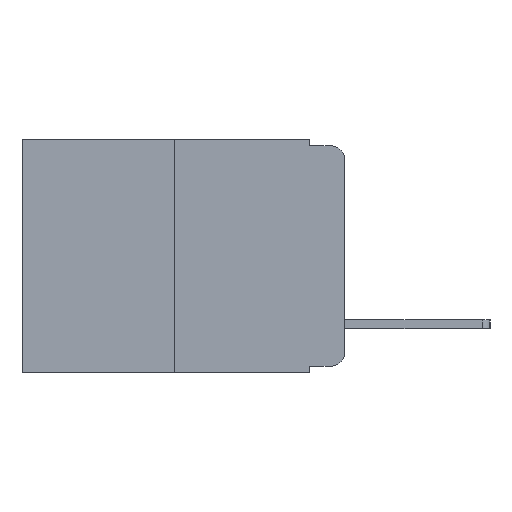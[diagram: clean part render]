
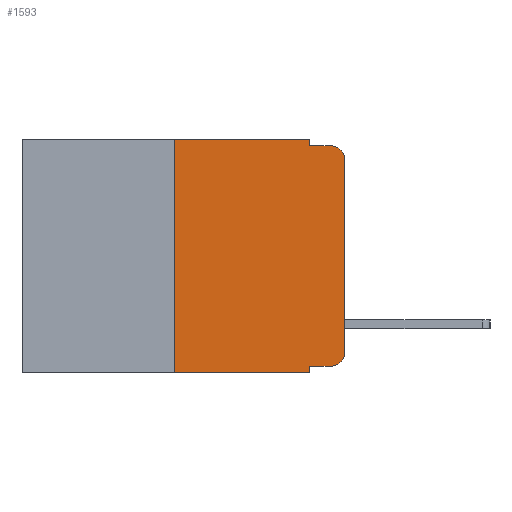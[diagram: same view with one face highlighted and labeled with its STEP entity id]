
A CAD part, left-side view. The second image highlights one B-rep face of the part: STEP entity #1593.
In plain terms, the highlighted planar face has unit normal (-1, 0, 0).
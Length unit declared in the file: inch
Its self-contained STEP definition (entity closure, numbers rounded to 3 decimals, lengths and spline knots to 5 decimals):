
#31 = CARTESIAN_POINT ( 'NONE',  ( 0., 0.02, -0.333 ) ) ;
#85 = EDGE_CURVE ( 'NONE', #5501, #1997, #14137, .T. ) ;
#293 = VECTOR ( 'NONE', #751, 39.37008 ) ;
#671 = VERTEX_POINT ( 'NONE', #8216 ) ;
#751 = DIRECTION ( 'NONE',  ( 0., 0., 1. ) ) ;
#843 = VERTEX_POINT ( 'NONE', #7158 ) ;
#1154 = AXIS2_PLACEMENT_3D ( 'NONE', #13537, #6124, #11229 ) ;
#1593 = ADVANCED_FACE ( 'NONE', ( #13270 ), #2182, .F. ) ;
#1685 = DIRECTION ( 'NONE',  ( 0., -1., 0. ) ) ;
#1717 = CARTESIAN_POINT ( 'NONE',  ( 0., 0.051, -0.01 ) ) ;
#1826 = VERTEX_POINT ( 'NONE', #7846 ) ;
#1928 = LINE ( 'NONE', #10556, #7609 ) ;
#1997 = VERTEX_POINT ( 'NONE', #6578 ) ;
#2041 = CARTESIAN_POINT ( 'NONE',  ( 0., 0., -0.03 ) ) ;
#2141 = DIRECTION ( 'NONE',  ( 0., 0., -1. ) ) ;
#2182 = PLANE ( 'NONE',  #2847 ) ;
#2289 = ORIENTED_EDGE ( 'NONE', *, *, #13253, .F. ) ;
#2492 = EDGE_CURVE ( 'NONE', #6378, #1997, #11757, .T. ) ;
#2517 = DIRECTION ( 'NONE',  ( 0., 0., -1. ) ) ;
#2654 = DIRECTION ( 'NONE',  ( 0., 0., -1. ) ) ;
#2658 = CIRCLE ( 'NONE', #13845, 0.02 ) ;
#2847 = AXIS2_PLACEMENT_3D ( 'NONE', #8989, #5387, #2517 ) ;
#3054 = CARTESIAN_POINT ( 'NONE',  ( 0., 0.051, -0.343 ) ) ;
#3188 = EDGE_CURVE ( 'NONE', #10214, #7503, #8926, .T. ) ;
#3283 = LINE ( 'NONE', #5036, #12225 ) ;
#3416 = ORIENTED_EDGE ( 'NONE', *, *, #5824, .T. ) ;
#3748 = CARTESIAN_POINT ( 'NONE',  ( 0., 0.25, -0.343 ) ) ;
#3804 = CARTESIAN_POINT ( 'NONE',  ( 0., 0.051, -0.333 ) ) ;
#3916 = DIRECTION ( 'NONE',  ( 0., 0., 1. ) ) ;
#4067 = EDGE_CURVE ( 'NONE', #13484, #6378, #3283, .T. ) ;
#4830 = DIRECTION ( 'NONE',  ( -1., 0., 0. ) ) ;
#5036 = CARTESIAN_POINT ( 'NONE',  ( 0., 0., 0. ) ) ;
#5387 = DIRECTION ( 'NONE',  ( 1., 0., 0. ) ) ;
#5501 = VERTEX_POINT ( 'NONE', #7856 ) ;
#5505 = VECTOR ( 'NONE', #12422, 39.37008 ) ;
#5591 = DIRECTION ( 'NONE',  ( 0., -1., 0. ) ) ;
#5633 = DIRECTION ( 'NONE',  ( 0., -1., 0. ) ) ;
#5701 = VECTOR ( 'NONE', #1685, 39.37008 ) ;
#5824 = EDGE_CURVE ( 'NONE', #6898, #13484, #2658, .T. ) ;
#5841 = LINE ( 'NONE', #6857, #5505 ) ;
#6124 = DIRECTION ( 'NONE',  ( -1., 0., 0. ) ) ;
#6128 = VECTOR ( 'NONE', #2141, 39.37008 ) ;
#6378 = VERTEX_POINT ( 'NONE', #2041 ) ;
#6498 = CARTESIAN_POINT ( 'NONE',  ( 0., 0., -0.313 ) ) ;
#6578 = CARTESIAN_POINT ( 'NONE',  ( 0., 0.02, -0.01 ) ) ;
#6857 = CARTESIAN_POINT ( 'NONE',  ( 0., 0.473, 0. ) ) ;
#6898 = VERTEX_POINT ( 'NONE', #31 ) ;
#7158 = CARTESIAN_POINT ( 'NONE',  ( 0., 0.25, 0. ) ) ;
#7234 = CARTESIAN_POINT ( 'NONE',  ( 0., 0.02, -0.313 ) ) ;
#7245 = ORIENTED_EDGE ( 'NONE', *, *, #85, .F. ) ;
#7308 = EDGE_CURVE ( 'NONE', #671, #6898, #12293, .T. ) ;
#7503 = VERTEX_POINT ( 'NONE', #3054 ) ;
#7609 = VECTOR ( 'NONE', #2654, 39.37008 ) ;
#7846 = CARTESIAN_POINT ( 'NONE',  ( 0., 0.051, 0. ) ) ;
#7856 = CARTESIAN_POINT ( 'NONE',  ( 0., 0.051, -0.01 ) ) ;
#7859 = ORIENTED_EDGE ( 'NONE', *, *, #7308, .T. ) ;
#8216 = CARTESIAN_POINT ( 'NONE',  ( 0., 0.051, -0.333 ) ) ;
#8238 = ORIENTED_EDGE ( 'NONE', *, *, #3188, .T. ) ;
#8489 = ORIENTED_EDGE ( 'NONE', *, *, #8826, .F. ) ;
#8826 = EDGE_CURVE ( 'NONE', #671, #7503, #12415, .T. ) ;
#8926 = LINE ( 'NONE', #11782, #14047 ) ;
#8989 = CARTESIAN_POINT ( 'NONE',  ( 0., 0.473, 0. ) ) ;
#9336 = VECTOR ( 'NONE', #5591, 39.37008 ) ;
#9781 = ORIENTED_EDGE ( 'NONE', *, *, #4067, .T. ) ;
#10198 = DIRECTION ( 'NONE',  ( 0., 0., -1. ) ) ;
#10214 = VERTEX_POINT ( 'NONE', #3748 ) ;
#10556 = CARTESIAN_POINT ( 'NONE',  ( 0., 0.051, 0. ) ) ;
#10626 = ORIENTED_EDGE ( 'NONE', *, *, #11837, .F. ) ;
#11229 = DIRECTION ( 'NONE',  ( 0., 0., -1. ) ) ;
#11757 = CIRCLE ( 'NONE', #1154, 0.02 ) ;
#11782 = CARTESIAN_POINT ( 'NONE',  ( 0., 0.473, -0.343 ) ) ;
#11837 = EDGE_CURVE ( 'NONE', #10214, #843, #12386, .T. ) ;
#12113 = ORIENTED_EDGE ( 'NONE', *, *, #2492, .T. ) ;
#12225 = VECTOR ( 'NONE', #3916, 39.37008 ) ;
#12243 = CARTESIAN_POINT ( 'NONE',  ( 0., 0.051, 0. ) ) ;
#12293 = LINE ( 'NONE', #3804, #9336 ) ;
#12386 = LINE ( 'NONE', #13122, #293 ) ;
#12415 = LINE ( 'NONE', #12243, #6128 ) ;
#12422 = DIRECTION ( 'NONE',  ( 0., -1., 0. ) ) ;
#12953 = EDGE_LOOP ( 'NONE', ( #9781, #12113, #7245, #2289, #13622, #10626, #8238, #8489, #7859, #3416 ) ) ;
#13122 = CARTESIAN_POINT ( 'NONE',  ( 0., 0.25, 0. ) ) ;
#13253 = EDGE_CURVE ( 'NONE', #1826, #5501, #1928, .T. ) ;
#13270 = FACE_OUTER_BOUND ( 'NONE', #12953, .T. ) ;
#13484 = VERTEX_POINT ( 'NONE', #6498 ) ;
#13537 = CARTESIAN_POINT ( 'NONE',  ( 0., 0.02, -0.03 ) ) ;
#13622 = ORIENTED_EDGE ( 'NONE', *, *, #14152, .F. ) ;
#13845 = AXIS2_PLACEMENT_3D ( 'NONE', #7234, #4830, #10198 ) ;
#14047 = VECTOR ( 'NONE', #5633, 39.37008 ) ;
#14137 = LINE ( 'NONE', #1717, #5701 ) ;
#14152 = EDGE_CURVE ( 'NONE', #843, #1826, #5841, .T. ) ;
